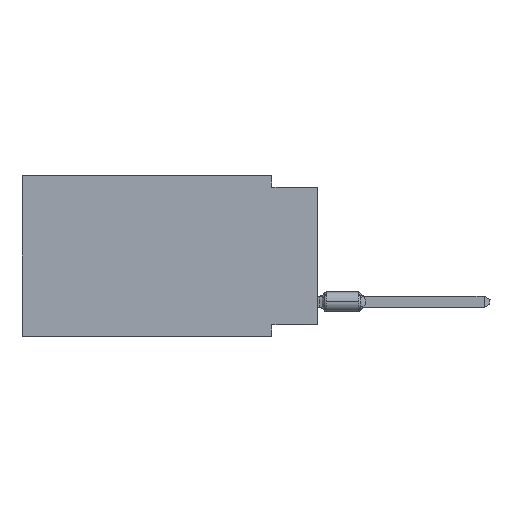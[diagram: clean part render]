
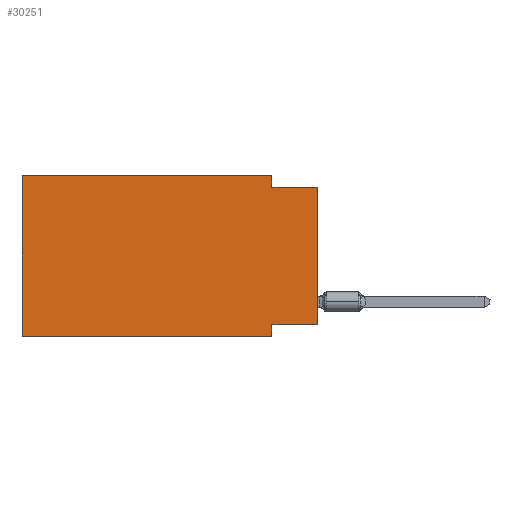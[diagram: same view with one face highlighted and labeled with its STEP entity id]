
A CAD part, left-side view. The second image highlights one B-rep face of the part: STEP entity #30251.
In plain terms, the highlighted planar face has unit normal (-1, 0, 0).
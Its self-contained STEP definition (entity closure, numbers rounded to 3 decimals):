
#2122 = LINE ( 'NONE', #49911, #37648 ) ;
#3896 = ORIENTED_EDGE ( 'NONE', *, *, #46814, .F. ) ;
#4389 = CARTESIAN_POINT ( 'NONE',  ( 0., 0., 0. ) ) ;
#5090 = CARTESIAN_POINT ( 'NONE',  ( 0., 0., -8.255 ) ) ;
#5510 = VERTEX_POINT ( 'NONE', #52573 ) ;
#5861 = EDGE_CURVE ( 'NONE', #52624, #14573, #12186, .T. ) ;
#6586 = CARTESIAN_POINT ( 'NONE',  ( 0., 2.54, -0.635 ) ) ;
#6987 = EDGE_CURVE ( 'NONE', #14573, #35007, #31840, .T. ) ;
#7119 = DIRECTION ( 'NONE',  ( 0., -1., 0. ) ) ;
#7834 = CARTESIAN_POINT ( 'NONE',  ( 0., 2.54, 0. ) ) ;
#7902 = ORIENTED_EDGE ( 'NONE', *, *, #54476, .F. ) ;
#10353 = VERTEX_POINT ( 'NONE', #42346 ) ;
#12186 = LINE ( 'NONE', #7834, #50262 ) ;
#14573 = VERTEX_POINT ( 'NONE', #6586 ) ;
#15854 = EDGE_LOOP ( 'NONE', ( #52054, #46716, #55106, #3896, #28572, #55254, #28041, #7902 ) ) ;
#18402 = CARTESIAN_POINT ( 'NONE',  ( 0., 0., -0.635 ) ) ;
#19715 = CARTESIAN_POINT ( 'NONE',  ( 0., 16.383, -8.89 ) ) ;
#20216 = LINE ( 'NONE', #28685, #45082 ) ;
#21131 = DIRECTION ( 'NONE',  ( 1., 0., 0. ) ) ;
#23354 = CARTESIAN_POINT ( 'NONE',  ( 0., 16.383, 0. ) ) ;
#24424 = DIRECTION ( 'NONE',  ( 0., 0., 1. ) ) ;
#27110 = DIRECTION ( 'NONE',  ( 0., 0., -1. ) ) ;
#27769 = VERTEX_POINT ( 'NONE', #19715 ) ;
#28041 = ORIENTED_EDGE ( 'NONE', *, *, #52079, .F. ) ;
#28181 = EDGE_CURVE ( 'NONE', #27769, #5510, #53183, .T. ) ;
#28572 = ORIENTED_EDGE ( 'NONE', *, *, #28181, .F. ) ;
#28685 = CARTESIAN_POINT ( 'NONE',  ( 0., 0., -8.255 ) ) ;
#29584 = VECTOR ( 'NONE', #33365, 1000. ) ;
#29917 = VERTEX_POINT ( 'NONE', #50245 ) ;
#30251 = ADVANCED_FACE ( 'NONE', ( #54574 ), #44902, .F. ) ;
#31203 = CARTESIAN_POINT ( 'NONE',  ( 0., 2.54, -8.89 ) ) ;
#31251 = DIRECTION ( 'NONE',  ( 0., 0., -1. ) ) ;
#31840 = LINE ( 'NONE', #18402, #51241 ) ;
#33365 = DIRECTION ( 'NONE',  ( 0., -1., 0. ) ) ;
#33850 = CARTESIAN_POINT ( 'NONE',  ( 0., 2.54, 0. ) ) ;
#34296 = DIRECTION ( 'NONE',  ( 0., 0., -1. ) ) ;
#35007 = VERTEX_POINT ( 'NONE', #53096 ) ;
#36484 = VECTOR ( 'NONE', #43435, 1000. ) ;
#36811 = LINE ( 'NONE', #31203, #41875 ) ;
#37648 = VECTOR ( 'NONE', #7119, 1000. ) ;
#38823 = CARTESIAN_POINT ( 'NONE',  ( 0., 16.383, 0. ) ) ;
#39309 = CARTESIAN_POINT ( 'NONE',  ( 0., 16.383, 0. ) ) ;
#41875 = VECTOR ( 'NONE', #27110, 1000. ) ;
#42346 = CARTESIAN_POINT ( 'NONE',  ( 0., 2.54, -8.89 ) ) ;
#43365 = DIRECTION ( 'NONE',  ( 0., 1., 0. ) ) ;
#43435 = DIRECTION ( 'NONE',  ( 0., 0., 1. ) ) ;
#44364 = AXIS2_PLACEMENT_3D ( 'NONE', #39309, #21131, #34296 ) ;
#44902 = PLANE ( 'NONE',  #44364 ) ;
#45082 = VECTOR ( 'NONE', #43365, 1000. ) ;
#46306 = EDGE_CURVE ( 'NONE', #50158, #35007, #53105, .T. ) ;
#46716 = ORIENTED_EDGE ( 'NONE', *, *, #6987, .F. ) ;
#46814 = EDGE_CURVE ( 'NONE', #5510, #52624, #49197, .T. ) ;
#49197 = LINE ( 'NONE', #23354, #29584 ) ;
#49911 = CARTESIAN_POINT ( 'NONE',  ( 0., 16.383, -8.89 ) ) ;
#50158 = VERTEX_POINT ( 'NONE', #5090 ) ;
#50245 = CARTESIAN_POINT ( 'NONE',  ( 0., 2.54, -8.255 ) ) ;
#50262 = VECTOR ( 'NONE', #31251, 1000. ) ;
#51193 = DIRECTION ( 'NONE',  ( 0., -1., 0. ) ) ;
#51241 = VECTOR ( 'NONE', #51193, 1000. ) ;
#52054 = ORIENTED_EDGE ( 'NONE', *, *, #46306, .T. ) ;
#52079 = EDGE_CURVE ( 'NONE', #29917, #10353, #36811, .T. ) ;
#52573 = CARTESIAN_POINT ( 'NONE',  ( 0., 16.383, 0. ) ) ;
#52624 = VERTEX_POINT ( 'NONE', #33850 ) ;
#53096 = CARTESIAN_POINT ( 'NONE',  ( 0., 0., -0.635 ) ) ;
#53105 = LINE ( 'NONE', #4389, #36484 ) ;
#53183 = LINE ( 'NONE', #38823, #53280 ) ;
#53280 = VECTOR ( 'NONE', #24424, 1000. ) ;
#54476 = EDGE_CURVE ( 'NONE', #50158, #29917, #20216, .T. ) ;
#54574 = FACE_OUTER_BOUND ( 'NONE', #15854, .T. ) ;
#55106 = ORIENTED_EDGE ( 'NONE', *, *, #5861, .F. ) ;
#55254 = ORIENTED_EDGE ( 'NONE', *, *, #60452, .T. ) ;
#60452 = EDGE_CURVE ( 'NONE', #27769, #10353, #2122, .T. ) ;
